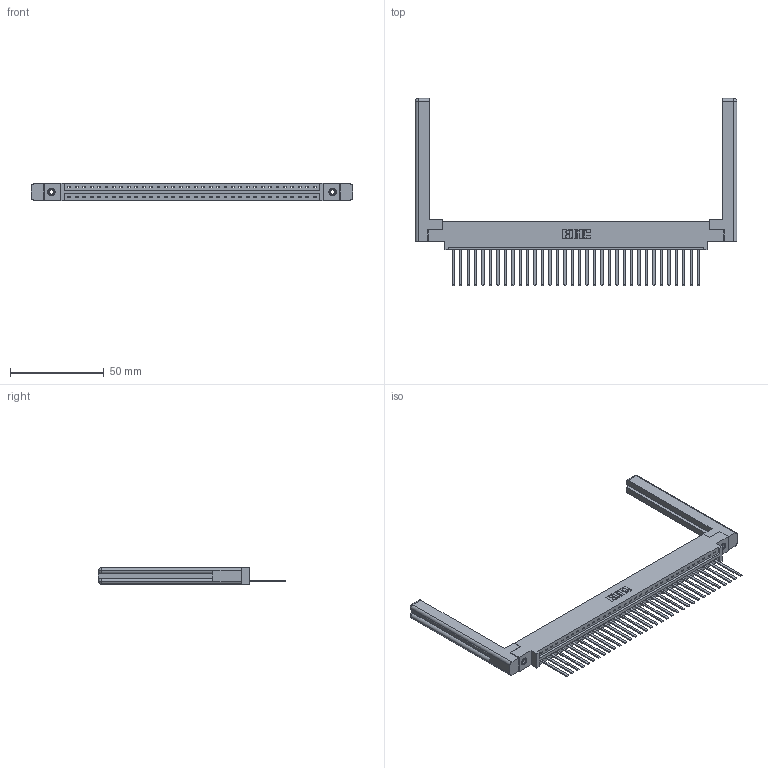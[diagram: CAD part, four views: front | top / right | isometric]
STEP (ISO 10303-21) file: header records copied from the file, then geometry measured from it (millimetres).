
FILE_DESCRIPTION (( 'STEP AP203' ), '1' );
FILE_NAME ('337-034-544-658.STEP', '2019-10-01T12:12:08', ( '' ), ( '' ), 'SwSTEP 2.0', 'SolidWorks 2016', '' );
FILE_SCHEMA (( 'CONFIG_CONTROL_DESIGN' ));
Length unit declared in the file: inch
Products named in the file (5): 307-220-058; 345-292-001_345-293-144; 337 Part_0.170 Offset - 0.156 Dia-TI; 337-034-544-658; 345-250-001_345-250-001-102
Assembly tree (39 placements, depth 2):
  337-034-544-658
    337 Part_0.170 Offset - 0.156 Dia-TI
    345-292-001_345-293-144  x34
    345-250-001_345-250-001-102  x2
    307-220-058  x2
Bounding box: 171.35 x 99.7 x 9.4 mm (x, y, z)
Volume: 25147.1 mm3; surface area: 25145.1 mm2
Topology: 39 solids, 39 shells, 2164 faces, 6457 edges, 4246 vertices
Faces by surface type: plane 1586, cylinder 554, cone 12, torus 12
Entity records: 28890 total; most frequent: CARTESIAN_POINT 5031, ORIENTED_EDGE 4940, DIRECTION 4266, EDGE_CURVE 2470, LINE 2298, VECTOR 2298, VERTEX_POINT 1638, AXIS2_PLACEMENT_3D 984
